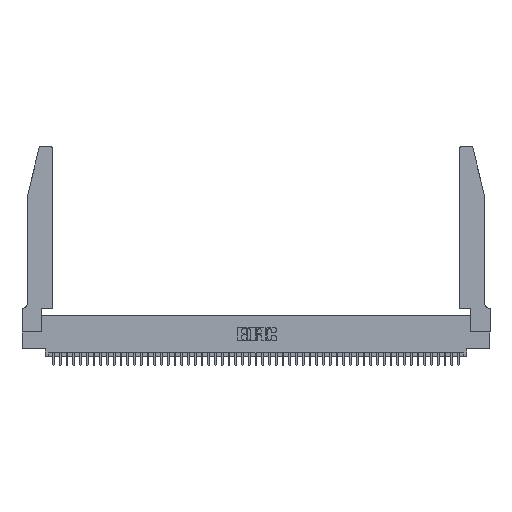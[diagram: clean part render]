
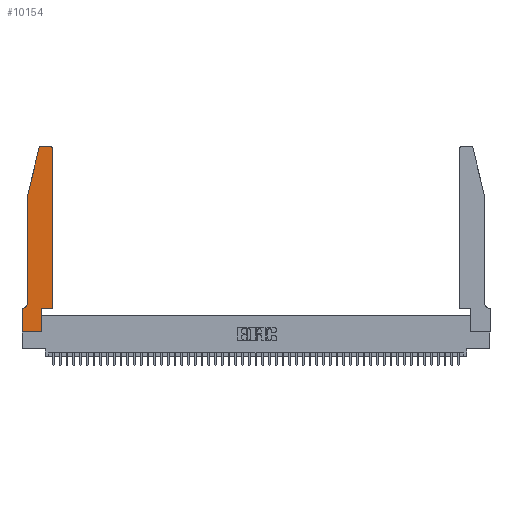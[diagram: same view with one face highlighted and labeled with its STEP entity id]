
A CAD part, top view. The second image highlights one B-rep face of the part: STEP entity #10154.
In plain terms, the highlighted planar face has unit normal (0, 0, 1).
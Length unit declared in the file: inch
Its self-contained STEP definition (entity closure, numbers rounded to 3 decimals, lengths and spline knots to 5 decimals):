
#222 = VERTEX_POINT ( 'NONE', #17879 ) ;
#836 = VERTEX_POINT ( 'NONE', #36810 ) ;
#1948 = CARTESIAN_POINT ( 'NONE',  ( 0.2865, 0.35, 0.37 ) ) ;
#2195 = ORIENTED_EDGE ( 'NONE', *, *, #48641, .T. ) ;
#2381 = CARTESIAN_POINT ( 'NONE',  ( 0.4205, 2.75, 0.37 ) ) ;
#2415 = DIRECTION ( 'NONE',  ( 1., 0., 0. ) ) ;
#2524 = EDGE_CURVE ( 'NONE', #222, #836, #4794, .T. ) ;
#3053 = CIRCLE ( 'NONE', #42493, 0.07 ) ;
#3181 = CARTESIAN_POINT ( 'NONE',  ( 0.25487, 2.72718, 0.37 ) ) ;
#3261 = CARTESIAN_POINT ( 'NONE',  ( 0.0755, 2., 0.37 ) ) ;
#3431 = VERTEX_POINT ( 'NONE', #3181 ) ;
#3598 = VECTOR ( 'NONE', #48322, 39.37008 ) ;
#3826 = DIRECTION ( 'NONE',  ( 1., 0., 0. ) ) ;
#4043 = EDGE_CURVE ( 'NONE', #30444, #35378, #47679, .T. ) ;
#4206 = CARTESIAN_POINT ( 'NONE',  ( 0.284, 2.75, 0.37 ) ) ;
#4423 = CARTESIAN_POINT ( 'NONE',  ( 0.2865, 0., 0.37 ) ) ;
#4794 = LINE ( 'NONE', #44455, #3598 ) ;
#4852 = ORIENTED_EDGE ( 'NONE', *, *, #7179, .T. ) ;
#5316 = VECTOR ( 'NONE', #49543, 39.37008 ) ;
#6262 = EDGE_CURVE ( 'NONE', #3431, #6944, #44542, .T. ) ;
#6873 = VECTOR ( 'NONE', #2415, 39.37008 ) ;
#6944 = VERTEX_POINT ( 'NONE', #30351 ) ;
#7179 = EDGE_CURVE ( 'NONE', #24969, #20230, #36079, .T. ) ;
#7247 = CARTESIAN_POINT ( 'NONE',  ( 0.0055, 0.42, 0.37 ) ) ;
#7512 = LINE ( 'NONE', #1948, #8718 ) ;
#8051 = CARTESIAN_POINT ( 'NONE',  ( 0.4505, 0.35, 0.37 ) ) ;
#8277 = CARTESIAN_POINT ( 'NONE',  ( 0., 0.35, 0.37 ) ) ;
#8718 = VECTOR ( 'NONE', #29132, 39.37008 ) ;
#9331 = VERTEX_POINT ( 'NONE', #30083 ) ;
#10154 = ADVANCED_FACE ( 'NONE', ( #31506 ), #42528, .T. ) ;
#10701 = ORIENTED_EDGE ( 'NONE', *, *, #2524, .T. ) ;
#11155 = DIRECTION ( 'NONE',  ( -1., 0., 0. ) ) ;
#11290 = CARTESIAN_POINT ( 'NONE',  ( 0.4205, 2.72, 0.37 ) ) ;
#12204 = AXIS2_PLACEMENT_3D ( 'NONE', #38493, #19321, #46404 ) ;
#12260 = ORIENTED_EDGE ( 'NONE', *, *, #36314, .T. ) ;
#12328 = DIRECTION ( 'NONE',  ( -1., 0., 0. ) ) ;
#12411 = AXIS2_PLACEMENT_3D ( 'NONE', #11290, #38426, #15204 ) ;
#12982 = VECTOR ( 'NONE', #12328, 39.37008 ) ;
#13364 = VERTEX_POINT ( 'NONE', #49252 ) ;
#13455 = EDGE_CURVE ( 'NONE', #9331, #30444, #3053, .T. ) ;
#14460 = LINE ( 'NONE', #22464, #5316 ) ;
#15204 = DIRECTION ( 'NONE',  ( 1., 0., 0. ) ) ;
#16299 = LINE ( 'NONE', #8051, #25427 ) ;
#17274 = ORIENTED_EDGE ( 'NONE', *, *, #4043, .T. ) ;
#17382 = VECTOR ( 'NONE', #31262, 39.37008 ) ;
#17730 = EDGE_CURVE ( 'NONE', #38320, #42438, #37841, .T. ) ;
#17879 = CARTESIAN_POINT ( 'NONE',  ( 0.2865, 0.35, 0.37 ) ) ;
#18600 = LINE ( 'NONE', #19717, #17382 ) ;
#18874 = DIRECTION ( 'NONE',  ( -0.239, -0.971, 0. ) ) ;
#19075 = DIRECTION ( 'NONE',  ( -1., 0., 0. ) ) ;
#19187 = ORIENTED_EDGE ( 'NONE', *, *, #6262, .T. ) ;
#19201 = EDGE_CURVE ( 'NONE', #20230, #3431, #39132, .T. ) ;
#19321 = DIRECTION ( 'NONE',  ( 0., 0., 1. ) ) ;
#19717 = CARTESIAN_POINT ( 'NONE',  ( 0., 0., 0.37 ) ) ;
#19763 = DIRECTION ( 'NONE',  ( 0., 1., 0. ) ) ;
#20230 = VERTEX_POINT ( 'NONE', #4206 ) ;
#20308 = ORIENTED_EDGE ( 'NONE', *, *, #19201, .T. ) ;
#20515 = EDGE_CURVE ( 'NONE', #42438, #222, #7512, .T. ) ;
#21171 = ORIENTED_EDGE ( 'NONE', *, *, #17730, .T. ) ;
#21756 = CIRCLE ( 'NONE', #12411, 0.03 ) ;
#22464 = CARTESIAN_POINT ( 'NONE',  ( 0.0755, 2., 0.37 ) ) ;
#23946 = VECTOR ( 'NONE', #18874, 39.37008 ) ;
#24969 = VERTEX_POINT ( 'NONE', #2381 ) ;
#25314 = ORIENTED_EDGE ( 'NONE', *, *, #13455, .T. ) ;
#25427 = VECTOR ( 'NONE', #19763, 39.37008 ) ;
#27090 = DIRECTION ( 'NONE',  ( 0., 0., 1. ) ) ;
#27149 = VECTOR ( 'NONE', #19075, 39.37008 ) ;
#29132 = DIRECTION ( 'NONE',  ( 0., 1., 0. ) ) ;
#29994 = EDGE_CURVE ( 'NONE', #35378, #38320, #18600, .T. ) ;
#30083 = CARTESIAN_POINT ( 'NONE',  ( 0.0755, 0.42, 0.37 ) ) ;
#30351 = CARTESIAN_POINT ( 'NONE',  ( 0.0755, 2., 0.37 ) ) ;
#30426 = ORIENTED_EDGE ( 'NONE', *, *, #29994, .T. ) ;
#30444 = VERTEX_POINT ( 'NONE', #38690 ) ;
#31262 = DIRECTION ( 'NONE',  ( 0., -1., 0. ) ) ;
#31301 = AXIS2_PLACEMENT_3D ( 'NONE', #50221, #27090, #3826 ) ;
#31506 = FACE_OUTER_BOUND ( 'NONE', #50135, .T. ) ;
#34385 = DIRECTION ( 'NONE',  ( 0., 0., -1. ) ) ;
#35378 = VERTEX_POINT ( 'NONE', #8277 ) ;
#36020 = EDGE_CURVE ( 'NONE', #836, #13364, #16299, .T. ) ;
#36079 = LINE ( 'NONE', #39464, #12982 ) ;
#36314 = EDGE_CURVE ( 'NONE', #6944, #9331, #14460, .T. ) ;
#36810 = CARTESIAN_POINT ( 'NONE',  ( 0.4505, 0.35, 0.37 ) ) ;
#37841 = LINE ( 'NONE', #48850, #6873 ) ;
#38320 = VERTEX_POINT ( 'NONE', #42538 ) ;
#38415 = CARTESIAN_POINT ( 'NONE',  ( 0.0755, 0.35, 0.37 ) ) ;
#38426 = DIRECTION ( 'NONE',  ( 0., 0., 1. ) ) ;
#38493 = CARTESIAN_POINT ( 'NONE',  ( 0., 0.35, 0.37 ) ) ;
#38690 = CARTESIAN_POINT ( 'NONE',  ( 0.0055, 0.35, 0.37 ) ) ;
#39132 = CIRCLE ( 'NONE', #31301, 0.03 ) ;
#39464 = CARTESIAN_POINT ( 'NONE',  ( 0.2605, 2.75, 0.37 ) ) ;
#40806 = ORIENTED_EDGE ( 'NONE', *, *, #36020, .T. ) ;
#42438 = VERTEX_POINT ( 'NONE', #4423 ) ;
#42493 = AXIS2_PLACEMENT_3D ( 'NONE', #7247, #34385, #11155 ) ;
#42528 = PLANE ( 'NONE',  #12204 ) ;
#42538 = CARTESIAN_POINT ( 'NONE',  ( 0., 0., 0.37 ) ) ;
#44455 = CARTESIAN_POINT ( 'NONE',  ( 0.4505, 0.35, 0.37 ) ) ;
#44542 = LINE ( 'NONE', #3261, #23946 ) ;
#46244 = ORIENTED_EDGE ( 'NONE', *, *, #20515, .T. ) ;
#46404 = DIRECTION ( 'NONE',  ( 1., 0., 0. ) ) ;
#47679 = LINE ( 'NONE', #38415, #27149 ) ;
#48322 = DIRECTION ( 'NONE',  ( 1., 0., 0. ) ) ;
#48641 = EDGE_CURVE ( 'NONE', #13364, #24969, #21756, .T. ) ;
#48850 = CARTESIAN_POINT ( 'NONE',  ( 0., 0., 0.37 ) ) ;
#49252 = CARTESIAN_POINT ( 'NONE',  ( 0.4505, 2.72, 0.37 ) ) ;
#49543 = DIRECTION ( 'NONE',  ( 0., -1., 0. ) ) ;
#50135 = EDGE_LOOP ( 'NONE', ( #4852, #20308, #19187, #12260, #25314, #17274, #30426, #21171, #46244, #10701, #40806, #2195 ) ) ;
#50221 = CARTESIAN_POINT ( 'NONE',  ( 0.284, 2.72, 0.37 ) ) ;
